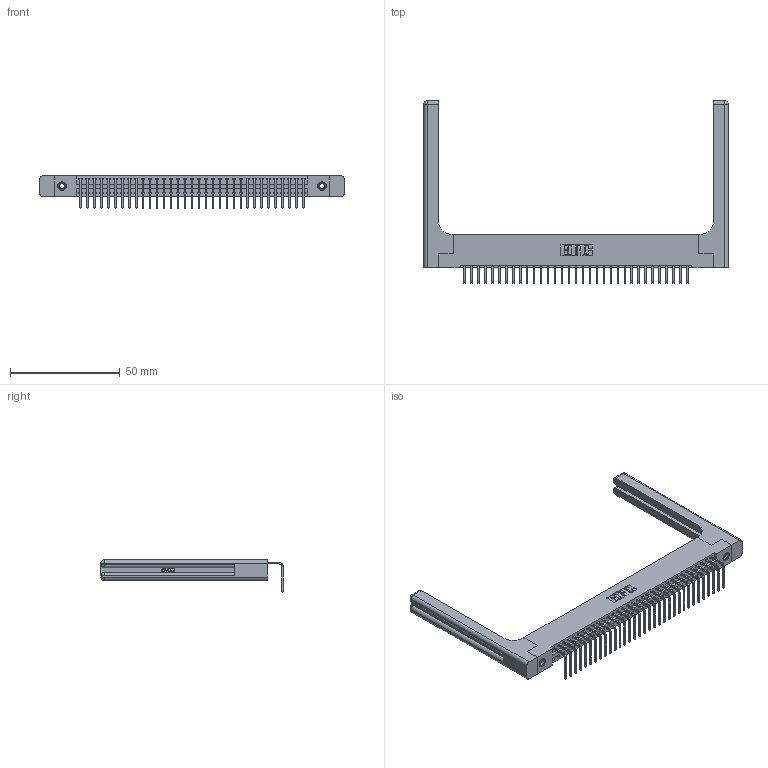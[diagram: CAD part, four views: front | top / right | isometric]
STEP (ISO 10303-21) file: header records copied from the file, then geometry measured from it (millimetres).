
FILE_DESCRIPTION (( 'STEP AP203' ), '1' );
FILE_NAME ('396-033-558-158.STEP', '2019-11-01T07:09:50', ( '' ), ( '' ), 'SwSTEP 2.0', 'SolidWorks 2016', '' );
FILE_SCHEMA (( 'CONFIG_CONTROL_DESIGN' ));
Length unit declared in the file: inch
Products named in the file (5): 345-250-001_345-250-001-102; 346-220-058_345-220-058; 396-033-558-158; 346 Part_Flush Mounting Lugs - 0.156 Dia-TH; 345-292-001_558 Tail - 2
Assembly tree (38 placements, depth 2):
  396-033-558-158
    346 Part_Flush Mounting Lugs - 0.156 Dia-TH
    345-292-001_558 Tail - 2  x33
    345-250-001_345-250-001-102  x2
    346-220-058_345-220-058  x2
Bounding box: 138.84 x 83.12 x 14.73 mm (x, y, z)
Volume: 20856 mm3; surface area: 22398.7 mm2
Topology: 38 solids, 38 shells, 2358 faces, 7001 edges, 4602 vertices
Faces by surface type: plane 1610, cylinder 688, bspline 36, cone 12, sphere 8, torus 4
Entity records: 26958 total; most frequent: CARTESIAN_POINT 5604, ORIENTED_EDGE 4368, DIRECTION 3886, EDGE_CURVE 2184, LINE 1828, VECTOR 1828, VERTEX_POINT 1446, AXIS2_PLACEMENT_3D 1029
